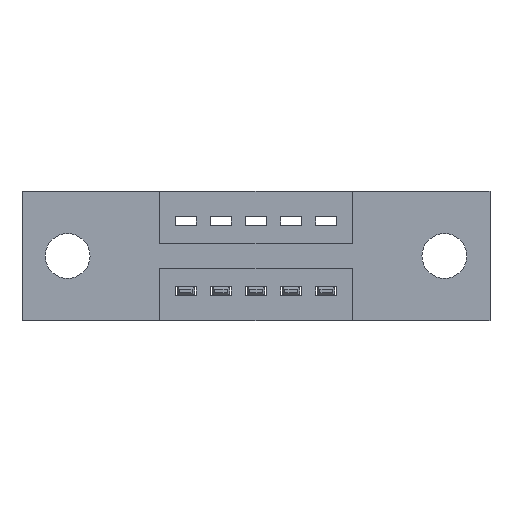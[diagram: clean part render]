
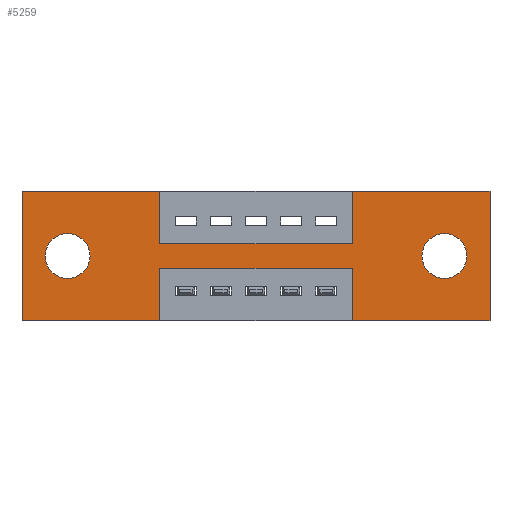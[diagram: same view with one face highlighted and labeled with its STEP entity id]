
A CAD part, front view. The second image highlights one B-rep face of the part: STEP entity #5259.
In plain terms, the highlighted planar face has unit normal (0, -1, 0).
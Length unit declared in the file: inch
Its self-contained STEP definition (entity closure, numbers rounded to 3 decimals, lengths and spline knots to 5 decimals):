
#45 = FACE_OUTER_BOUND ( 'NONE', #1583, .T. ) ;
#92 = VERTEX_POINT ( 'NONE', #8119 ) ;
#126 = DIRECTION ( 'NONE',  ( 1., 0., 0. ) ) ;
#144 = CARTESIAN_POINT ( 'NONE',  ( 0.13, 0., -0.185 ) ) ;
#170 = EDGE_CURVE ( 'NONE', #92, #7494, #3343, .T. ) ;
#172 = ORIENTED_EDGE ( 'NONE', *, *, #5071, .F. ) ;
#173 = VECTOR ( 'NONE', #1642, 39.37008 ) ;
#237 = CARTESIAN_POINT ( 'NONE',  ( 0., 0., -0.37 ) ) ;
#241 = ORIENTED_EDGE ( 'NONE', *, *, #170, .F. ) ;
#327 = EDGE_CURVE ( 'NONE', #2840, #2952, #4684, .T. ) ;
#359 = CARTESIAN_POINT ( 'NONE',  ( 0.3925, 0., -0.15 ) ) ;
#419 = ORIENTED_EDGE ( 'NONE', *, *, #8085, .T. ) ;
#454 = CARTESIAN_POINT ( 'NONE',  ( 0.3925, 0., -0.37 ) ) ;
#492 = DIRECTION ( 'NONE',  ( 0., 1., 0. ) ) ;
#553 = VECTOR ( 'NONE', #6925, 39.37008 ) ;
#561 = VECTOR ( 'NONE', #839, 39.37008 ) ;
#567 = EDGE_CURVE ( 'NONE', #8054, #92, #4392, .T. ) ;
#643 = ORIENTED_EDGE ( 'NONE', *, *, #6963, .T. ) ;
#696 = CARTESIAN_POINT ( 'NONE',  ( 0.3925, 0., 0. ) ) ;
#716 = AXIS2_PLACEMENT_3D ( 'NONE', #3739, #1792, #8342 ) ;
#767 = ORIENTED_EDGE ( 'NONE', *, *, #2496, .F. ) ;
#775 = LINE ( 'NONE', #4112, #1597 ) ;
#789 = DIRECTION ( 'NONE',  ( 1., 0., 0. ) ) ;
#839 = DIRECTION ( 'NONE',  ( 0., 0., 1. ) ) ;
#954 = LINE ( 'NONE', #4853, #561 ) ;
#992 = CARTESIAN_POINT ( 'NONE',  ( 0.9425, 0., -0.37 ) ) ;
#1121 = DIRECTION ( 'NONE',  ( 0., 0., 1. ) ) ;
#1190 = VECTOR ( 'NONE', #6714, 39.37008 ) ;
#1528 = DIRECTION ( 'NONE',  ( 0., 0., -1. ) ) ;
#1583 = EDGE_LOOP ( 'NONE', ( #4803, #767, #5571, #1745, #7183, #1812, #3202, #7880, #1863, #172, #241, #6926 ) ) ;
#1597 = VECTOR ( 'NONE', #126, 39.37008 ) ;
#1600 = CIRCLE ( 'NONE', #6443, 0.064 ) ;
#1642 = DIRECTION ( 'NONE',  ( 0., 0., -1. ) ) ;
#1667 = DIRECTION ( 'NONE',  ( 0., 0., -1. ) ) ;
#1687 = VERTEX_POINT ( 'NONE', #4258 ) ;
#1745 = ORIENTED_EDGE ( 'NONE', *, *, #8184, .F. ) ;
#1756 = CARTESIAN_POINT ( 'NONE',  ( 1.335, 0., 0. ) ) ;
#1792 = DIRECTION ( 'NONE',  ( 0., -1., 0. ) ) ;
#1806 = LINE ( 'NONE', #8402, #8418 ) ;
#1812 = ORIENTED_EDGE ( 'NONE', *, *, #4796, .F. ) ;
#1856 = DIRECTION ( 'NONE',  ( 0., 1., 0. ) ) ;
#1863 = ORIENTED_EDGE ( 'NONE', *, *, #7676, .F. ) ;
#1931 = CARTESIAN_POINT ( 'NONE',  ( 1.335, 0., -0.37 ) ) ;
#1951 = CIRCLE ( 'NONE', #5224, 0.064 ) ;
#2136 = LINE ( 'NONE', #4335, #173 ) ;
#2241 = CARTESIAN_POINT ( 'NONE',  ( 0.3925, 0., -0.22 ) ) ;
#2459 = CARTESIAN_POINT ( 'NONE',  ( 1.205, 0., -0.185 ) ) ;
#2471 = CARTESIAN_POINT ( 'NONE',  ( 0., 0., 0. ) ) ;
#2496 = EDGE_CURVE ( 'NONE', #8572, #7212, #3617, .T. ) ;
#2628 = CIRCLE ( 'NONE', #4974, 0.064 ) ;
#2676 = CARTESIAN_POINT ( 'NONE',  ( 0.9425, 0., -0.15 ) ) ;
#2714 = CARTESIAN_POINT ( 'NONE',  ( 0., 0., -0.37 ) ) ;
#2840 = VERTEX_POINT ( 'NONE', #8368 ) ;
#2902 = VERTEX_POINT ( 'NONE', #1756 ) ;
#2946 = EDGE_CURVE ( 'NONE', #7660, #7466, #1951, .T. ) ;
#2952 = VERTEX_POINT ( 'NONE', #7781 ) ;
#3202 = ORIENTED_EDGE ( 'NONE', *, *, #6059, .F. ) ;
#3343 = LINE ( 'NONE', #7377, #7073 ) ;
#3383 = EDGE_CURVE ( 'NONE', #7212, #8054, #6594, .T. ) ;
#3509 = DIRECTION ( 'NONE',  ( 0., 0., 1. ) ) ;
#3569 = LINE ( 'NONE', #237, #553 ) ;
#3585 = DIRECTION ( 'NONE',  ( -1., 0., 0. ) ) ;
#3617 = LINE ( 'NONE', #2241, #4557 ) ;
#3651 = ORIENTED_EDGE ( 'NONE', *, *, #327, .T. ) ;
#3739 = CARTESIAN_POINT ( 'NONE',  ( 0., 0., -0.37 ) ) ;
#3770 = DIRECTION ( 'NONE',  ( 0., 1., 0. ) ) ;
#3793 = CARTESIAN_POINT ( 'NONE',  ( 0.13, 0., -0.185 ) ) ;
#3810 = DIRECTION ( 'NONE',  ( 0., 0., -1. ) ) ;
#4025 = EDGE_LOOP ( 'NONE', ( #4600, #419 ) ) ;
#4067 = CARTESIAN_POINT ( 'NONE',  ( 0.3925, 0., -0.37 ) ) ;
#4112 = CARTESIAN_POINT ( 'NONE',  ( 0., 0., 0. ) ) ;
#4193 = CARTESIAN_POINT ( 'NONE',  ( 0.13, 0., -0.121 ) ) ;
#4258 = CARTESIAN_POINT ( 'NONE',  ( 0.3925, 0., 0. ) ) ;
#4273 = VERTEX_POINT ( 'NONE', #2676 ) ;
#4335 = CARTESIAN_POINT ( 'NONE',  ( 1.335, 0., 0. ) ) ;
#4392 = LINE ( 'NONE', #2714, #5528 ) ;
#4557 = VECTOR ( 'NONE', #3585, 39.37008 ) ;
#4600 = ORIENTED_EDGE ( 'NONE', *, *, #2946, .T. ) ;
#4684 = CIRCLE ( 'NONE', #6433, 0.064 ) ;
#4717 = DIRECTION ( 'NONE',  ( -1., 0., 0. ) ) ;
#4732 = DIRECTION ( 'NONE',  ( 0., 0., 1. ) ) ;
#4789 = DIRECTION ( 'NONE',  ( 0., 1., 0. ) ) ;
#4796 = EDGE_CURVE ( 'NONE', #7959, #2902, #775, .T. ) ;
#4803 = ORIENTED_EDGE ( 'NONE', *, *, #3383, .F. ) ;
#4853 = CARTESIAN_POINT ( 'NONE',  ( 0.9425, 0., -0.37 ) ) ;
#4974 = AXIS2_PLACEMENT_3D ( 'NONE', #144, #4789, #4732 ) ;
#5016 = LINE ( 'NONE', #8282, #7694 ) ;
#5071 = EDGE_CURVE ( 'NONE', #7494, #1687, #5665, .T. ) ;
#5146 = FACE_BOUND ( 'NONE', #4025, .T. ) ;
#5181 = VERTEX_POINT ( 'NONE', #359 ) ;
#5224 = AXIS2_PLACEMENT_3D ( 'NONE', #3793, #492, #1121 ) ;
#5255 = VECTOR ( 'NONE', #789, 39.37008 ) ;
#5257 = EDGE_CURVE ( 'NONE', #5181, #4273, #1806, .T. ) ;
#5259 = ADVANCED_FACE ( 'NONE', ( #6889, #5146, #45 ), #5747, .T. ) ;
#5526 = CARTESIAN_POINT ( 'NONE',  ( 0., 0., 0. ) ) ;
#5528 = VECTOR ( 'NONE', #4717, 39.37008 ) ;
#5571 = ORIENTED_EDGE ( 'NONE', *, *, #7875, .F. ) ;
#5615 = CARTESIAN_POINT ( 'NONE',  ( 0.9425, 0., 0. ) ) ;
#5665 = LINE ( 'NONE', #5526, #5255 ) ;
#5747 = PLANE ( 'NONE',  #716 ) ;
#5969 = EDGE_LOOP ( 'NONE', ( #643, #3651 ) ) ;
#6059 = EDGE_CURVE ( 'NONE', #4273, #7959, #5016, .T. ) ;
#6067 = VERTEX_POINT ( 'NONE', #992 ) ;
#6366 = EDGE_CURVE ( 'NONE', #2902, #8271, #2136, .T. ) ;
#6433 = AXIS2_PLACEMENT_3D ( 'NONE', #2459, #3770, #1667 ) ;
#6443 = AXIS2_PLACEMENT_3D ( 'NONE', #8470, #1856, #3810 ) ;
#6497 = CARTESIAN_POINT ( 'NONE',  ( 0.9425, 0., -0.22 ) ) ;
#6594 = LINE ( 'NONE', #4067, #1190 ) ;
#6714 = DIRECTION ( 'NONE',  ( 0., 0., -1. ) ) ;
#6775 = VECTOR ( 'NONE', #1528, 39.37008 ) ;
#6889 = FACE_BOUND ( 'NONE', #5969, .T. ) ;
#6925 = DIRECTION ( 'NONE',  ( -1., 0., 0. ) ) ;
#6926 = ORIENTED_EDGE ( 'NONE', *, *, #567, .F. ) ;
#6963 = EDGE_CURVE ( 'NONE', #2952, #2840, #1600, .T. ) ;
#7073 = VECTOR ( 'NONE', #3509, 39.37008 ) ;
#7183 = ORIENTED_EDGE ( 'NONE', *, *, #6366, .F. ) ;
#7212 = VERTEX_POINT ( 'NONE', #7530 ) ;
#7287 = LINE ( 'NONE', #696, #6775 ) ;
#7377 = CARTESIAN_POINT ( 'NONE',  ( 0., 0., 0. ) ) ;
#7466 = VERTEX_POINT ( 'NONE', #8384 ) ;
#7494 = VERTEX_POINT ( 'NONE', #2471 ) ;
#7530 = CARTESIAN_POINT ( 'NONE',  ( 0.3925, 0., -0.22 ) ) ;
#7660 = VERTEX_POINT ( 'NONE', #4193 ) ;
#7676 = EDGE_CURVE ( 'NONE', #1687, #5181, #7287, .T. ) ;
#7694 = VECTOR ( 'NONE', #8317, 39.37008 ) ;
#7696 = DIRECTION ( 'NONE',  ( 1., 0., 0. ) ) ;
#7781 = CARTESIAN_POINT ( 'NONE',  ( 1.205, 0., -0.121 ) ) ;
#7875 = EDGE_CURVE ( 'NONE', #6067, #8572, #954, .T. ) ;
#7880 = ORIENTED_EDGE ( 'NONE', *, *, #5257, .F. ) ;
#7959 = VERTEX_POINT ( 'NONE', #5615 ) ;
#8054 = VERTEX_POINT ( 'NONE', #454 ) ;
#8085 = EDGE_CURVE ( 'NONE', #7466, #7660, #2628, .T. ) ;
#8119 = CARTESIAN_POINT ( 'NONE',  ( 0., 0., -0.37 ) ) ;
#8184 = EDGE_CURVE ( 'NONE', #8271, #6067, #3569, .T. ) ;
#8271 = VERTEX_POINT ( 'NONE', #1931 ) ;
#8282 = CARTESIAN_POINT ( 'NONE',  ( 0.9425, 0., 0. ) ) ;
#8317 = DIRECTION ( 'NONE',  ( 0., 0., 1. ) ) ;
#8342 = DIRECTION ( 'NONE',  ( 0., 0., -1. ) ) ;
#8368 = CARTESIAN_POINT ( 'NONE',  ( 1.205, 0., -0.249 ) ) ;
#8384 = CARTESIAN_POINT ( 'NONE',  ( 0.13, 0., -0.249 ) ) ;
#8402 = CARTESIAN_POINT ( 'NONE',  ( 0.3925, 0., -0.15 ) ) ;
#8418 = VECTOR ( 'NONE', #7696, 39.37008 ) ;
#8470 = CARTESIAN_POINT ( 'NONE',  ( 1.205, 0., -0.185 ) ) ;
#8572 = VERTEX_POINT ( 'NONE', #6497 ) ;
